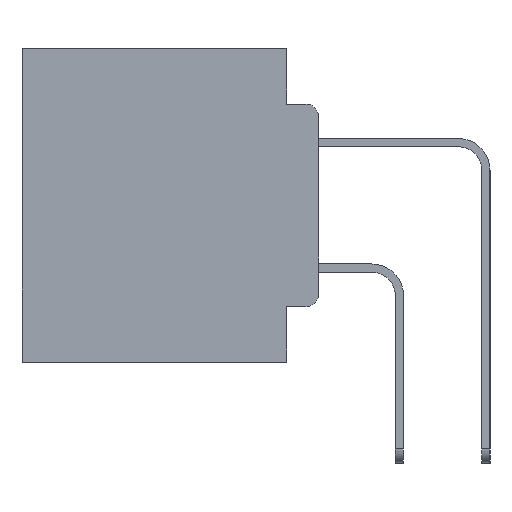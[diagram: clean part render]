
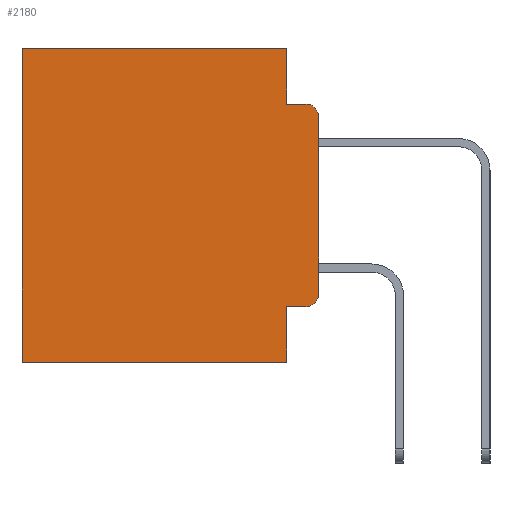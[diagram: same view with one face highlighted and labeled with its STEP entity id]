
A CAD part, left-side view. The second image highlights one B-rep face of the part: STEP entity #2180.
In plain terms, the highlighted planar face has unit normal (-1, 0, 0).
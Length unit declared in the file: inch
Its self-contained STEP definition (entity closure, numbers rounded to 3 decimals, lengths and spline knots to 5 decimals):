
#475 = EDGE_CURVE ( 'NONE', #26258, #29091, #3384, .T. ) ;
#726 = CARTESIAN_POINT ( 'NONE',  ( 0.298, 0.02, -0.3915 ) ) ;
#1034 = FACE_OUTER_BOUND ( 'NONE', #12781, .T. ) ;
#1204 = LINE ( 'NONE', #15353, #20089 ) ;
#1425 = DIRECTION ( 'NONE',  ( 0., 1., 0. ) ) ;
#1442 = AXIS2_PLACEMENT_3D ( 'NONE', #1560, #18130, #3938 ) ;
#1560 = CARTESIAN_POINT ( 'NONE',  ( 0.298, 0.02, -0.1085 ) ) ;
#2069 = EDGE_CURVE ( 'NONE', #15132, #26258, #16620, .T. ) ;
#2180 = ADVANCED_FACE ( 'NONE', ( #1034 ), #26045, .F. ) ;
#2286 = LINE ( 'NONE', #27553, #26651 ) ;
#2492 = VECTOR ( 'NONE', #11154, 39.37008 ) ;
#3110 = DIRECTION ( 'NONE',  ( 0., 0., -1. ) ) ;
#3175 = VERTEX_POINT ( 'NONE', #17423 ) ;
#3271 = CARTESIAN_POINT ( 'NONE',  ( 0.298, 0.051, -0.5 ) ) ;
#3384 = CIRCLE ( 'NONE', #5758, 0.02 ) ;
#3938 = DIRECTION ( 'NONE',  ( 0., 0., -1. ) ) ;
#4063 = EDGE_CURVE ( 'NONE', #12718, #3175, #18004, .T. ) ;
#4371 = CARTESIAN_POINT ( 'NONE',  ( 0.298, 0.051, -0.4115 ) ) ;
#4382 = CARTESIAN_POINT ( 'NONE',  ( 0.298, 0.051, -0.0885 ) ) ;
#5232 = EDGE_CURVE ( 'NONE', #15132, #12718, #8985, .T. ) ;
#5758 = AXIS2_PLACEMENT_3D ( 'NONE', #726, #17306, #3110 ) ;
#5912 = VECTOR ( 'NONE', #16276, 39.37008 ) ;
#6989 = LINE ( 'NONE', #28555, #25858 ) ;
#7509 = ORIENTED_EDGE ( 'NONE', *, *, #22705, .F. ) ;
#8170 = CARTESIAN_POINT ( 'NONE',  ( 0.298, 0.02, -0.4115 ) ) ;
#8247 = VECTOR ( 'NONE', #29321, 39.37008 ) ;
#8707 = ORIENTED_EDGE ( 'NONE', *, *, #5232, .F. ) ;
#8745 = LINE ( 'NONE', #22965, #2492 ) ;
#8985 = LINE ( 'NONE', #12989, #8247 ) ;
#9883 = CARTESIAN_POINT ( 'NONE',  ( 0.298, 0.02, -0.0885 ) ) ;
#10201 = VECTOR ( 'NONE', #1425, 39.37008 ) ;
#10918 = VERTEX_POINT ( 'NONE', #30318 ) ;
#11154 = DIRECTION ( 'NONE',  ( 0., 0., -1. ) ) ;
#11605 = EDGE_CURVE ( 'NONE', #10918, #3175, #1204, .T. ) ;
#11780 = ORIENTED_EDGE ( 'NONE', *, *, #4063, .F. ) ;
#12178 = DIRECTION ( 'NONE',  ( 0., 0., -1. ) ) ;
#12486 = ORIENTED_EDGE ( 'NONE', *, *, #2069, .T. ) ;
#12718 = VERTEX_POINT ( 'NONE', #3271 ) ;
#12781 = EDGE_LOOP ( 'NONE', ( #7509, #27823, #19423, #20537, #27136, #16907, #11780, #8707, #12486, #22822 ) ) ;
#12989 = CARTESIAN_POINT ( 'NONE',  ( 0.298, 0.051, 0. ) ) ;
#13220 = EDGE_CURVE ( 'NONE', #30084, #19021, #6989, .T. ) ;
#14345 = DIRECTION ( 'NONE',  ( 0., 0., -1. ) ) ;
#14417 = CARTESIAN_POINT ( 'NONE',  ( 0.298, 0., -0.3915 ) ) ;
#14794 = EDGE_CURVE ( 'NONE', #19021, #29817, #2286, .T. ) ;
#15132 = VERTEX_POINT ( 'NONE', #17119 ) ;
#15353 = CARTESIAN_POINT ( 'NONE',  ( 0.298, 0.473, 0. ) ) ;
#15600 = EDGE_CURVE ( 'NONE', #30084, #10918, #30156, .T. ) ;
#16276 = DIRECTION ( 'NONE',  ( 0., 1., 0. ) ) ;
#16620 = LINE ( 'NONE', #4371, #28306 ) ;
#16907 = ORIENTED_EDGE ( 'NONE', *, *, #11605, .T. ) ;
#17119 = CARTESIAN_POINT ( 'NONE',  ( 0.298, 0.051, -0.4115 ) ) ;
#17306 = DIRECTION ( 'NONE',  ( -1., 0., 0. ) ) ;
#17423 = CARTESIAN_POINT ( 'NONE',  ( 0.298, 0.473, -0.5 ) ) ;
#18004 = LINE ( 'NONE', #24876, #10201 ) ;
#18130 = DIRECTION ( 'NONE',  ( -1., 0., 0. ) ) ;
#19021 = VERTEX_POINT ( 'NONE', #4382 ) ;
#19423 = ORIENTED_EDGE ( 'NONE', *, *, #14794, .F. ) ;
#19524 = EDGE_CURVE ( 'NONE', #26974, #29817, #19753, .T. ) ;
#19753 = CIRCLE ( 'NONE', #1442, 0.02 ) ;
#20089 = VECTOR ( 'NONE', #29339, 39.37008 ) ;
#20327 = CARTESIAN_POINT ( 'NONE',  ( 0.298, 0.051, 0. ) ) ;
#20537 = ORIENTED_EDGE ( 'NONE', *, *, #13220, .F. ) ;
#21341 = CARTESIAN_POINT ( 'NONE',  ( 0.298, 0., 0. ) ) ;
#21892 = AXIS2_PLACEMENT_3D ( 'NONE', #21341, #28345, #14345 ) ;
#22705 = EDGE_CURVE ( 'NONE', #26974, #29091, #8745, .T. ) ;
#22822 = ORIENTED_EDGE ( 'NONE', *, *, #475, .T. ) ;
#22965 = CARTESIAN_POINT ( 'NONE',  ( 0.298, 0., 0. ) ) ;
#24876 = CARTESIAN_POINT ( 'NONE',  ( 0.298, 0., -0.5 ) ) ;
#24987 = CARTESIAN_POINT ( 'NONE',  ( 0.298, 0., -0.1085 ) ) ;
#25641 = DIRECTION ( 'NONE',  ( 0., -1., 0. ) ) ;
#25858 = VECTOR ( 'NONE', #12178, 39.37008 ) ;
#26045 = PLANE ( 'NONE',  #21892 ) ;
#26258 = VERTEX_POINT ( 'NONE', #8170 ) ;
#26651 = VECTOR ( 'NONE', #29846, 39.37008 ) ;
#26974 = VERTEX_POINT ( 'NONE', #24987 ) ;
#27136 = ORIENTED_EDGE ( 'NONE', *, *, #15600, .T. ) ;
#27553 = CARTESIAN_POINT ( 'NONE',  ( 0.298, 0.051, -0.0885 ) ) ;
#27823 = ORIENTED_EDGE ( 'NONE', *, *, #19524, .T. ) ;
#28011 = CARTESIAN_POINT ( 'NONE',  ( 0.298, 0., 0. ) ) ;
#28306 = VECTOR ( 'NONE', #25641, 39.37008 ) ;
#28345 = DIRECTION ( 'NONE',  ( 1., 0., 0. ) ) ;
#28555 = CARTESIAN_POINT ( 'NONE',  ( 0.298, 0.051, 0. ) ) ;
#29091 = VERTEX_POINT ( 'NONE', #14417 ) ;
#29321 = DIRECTION ( 'NONE',  ( 0., 0., -1. ) ) ;
#29339 = DIRECTION ( 'NONE',  ( 0., 0., -1. ) ) ;
#29817 = VERTEX_POINT ( 'NONE', #9883 ) ;
#29846 = DIRECTION ( 'NONE',  ( 0., -1., 0. ) ) ;
#30084 = VERTEX_POINT ( 'NONE', #20327 ) ;
#30156 = LINE ( 'NONE', #28011, #5912 ) ;
#30318 = CARTESIAN_POINT ( 'NONE',  ( 0.298, 0.473, 0. ) ) ;
